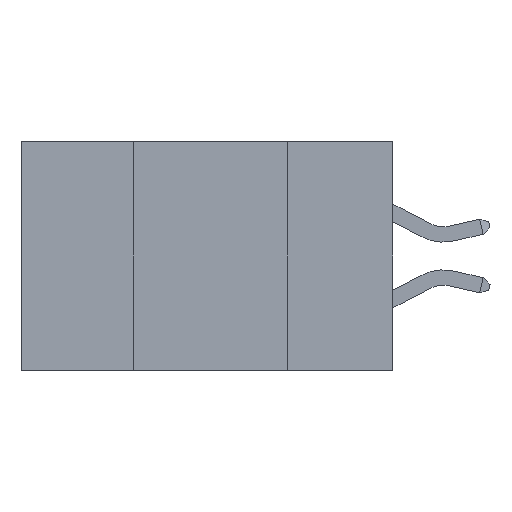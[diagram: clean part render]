
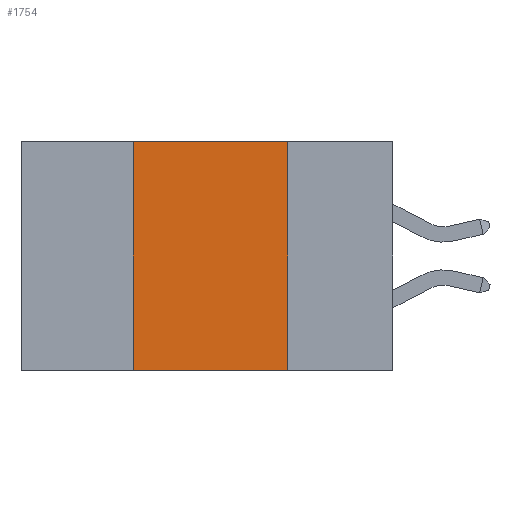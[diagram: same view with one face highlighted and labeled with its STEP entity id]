
A CAD part, left-side view. The second image highlights one B-rep face of the part: STEP entity #1754.
In plain terms, the highlighted planar face has unit normal (-1, 0, 0).
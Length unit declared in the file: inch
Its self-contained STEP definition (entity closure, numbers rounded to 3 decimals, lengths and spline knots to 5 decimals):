
#548 = VERTEX_POINT ( 'NONE', #22426 ) ;
#1312 = VERTEX_POINT ( 'NONE', #13641 ) ;
#1754 = ADVANCED_FACE ( 'NONE', ( #19253 ), #16965, .F. ) ;
#1822 = LINE ( 'NONE', #13468, #23692 ) ;
#3491 = ORIENTED_EDGE ( 'NONE', *, *, #4178, .T. ) ;
#3671 = DIRECTION ( 'NONE',  ( 1., 0., 0. ) ) ;
#3933 = ORIENTED_EDGE ( 'NONE', *, *, #21550, .F. ) ;
#4178 = EDGE_CURVE ( 'NONE', #20397, #548, #6258, .T. ) ;
#4592 = CARTESIAN_POINT ( 'NONE',  ( 0., 0.6, 0. ) ) ;
#5286 = EDGE_LOOP ( 'NONE', ( #19949, #3933, #6176, #3491 ) ) ;
#6176 = ORIENTED_EDGE ( 'NONE', *, *, #24717, .F. ) ;
#6258 = LINE ( 'NONE', #22367, #27716 ) ;
#7966 = DIRECTION ( 'NONE',  ( 0., 0., -1. ) ) ;
#8529 = LINE ( 'NONE', #18226, #10620 ) ;
#10620 = VECTOR ( 'NONE', #20649, 39.37008 ) ;
#11295 = DIRECTION ( 'NONE',  ( 0., -1., 0. ) ) ;
#13468 = CARTESIAN_POINT ( 'NONE',  ( 0., 0.42, 0. ) ) ;
#13641 = CARTESIAN_POINT ( 'NONE',  ( 0., 0.17, 0. ) ) ;
#13705 = CARTESIAN_POINT ( 'NONE',  ( 0., 0.42, -0.37 ) ) ;
#14936 = CARTESIAN_POINT ( 'NONE',  ( 0., 0.6, 0. ) ) ;
#16347 = VECTOR ( 'NONE', #11295, 39.37008 ) ;
#16682 = VERTEX_POINT ( 'NONE', #16713 ) ;
#16713 = CARTESIAN_POINT ( 'NONE',  ( 0., 0.42, 0. ) ) ;
#16965 = PLANE ( 'NONE',  #17863 ) ;
#17863 = AXIS2_PLACEMENT_3D ( 'NONE', #14936, #3671, #7966 ) ;
#18226 = CARTESIAN_POINT ( 'NONE',  ( 0., 0.17, 0. ) ) ;
#19253 = FACE_OUTER_BOUND ( 'NONE', #5286, .T. ) ;
#19949 = ORIENTED_EDGE ( 'NONE', *, *, #23741, .F. ) ;
#20397 = VERTEX_POINT ( 'NONE', #13705 ) ;
#20431 = DIRECTION ( 'NONE',  ( 0., 0., 1. ) ) ;
#20649 = DIRECTION ( 'NONE',  ( 0., 0., -1. ) ) ;
#21550 = EDGE_CURVE ( 'NONE', #16682, #1312, #24272, .T. ) ;
#22367 = CARTESIAN_POINT ( 'NONE',  ( 0., 0.6, -0.37 ) ) ;
#22426 = CARTESIAN_POINT ( 'NONE',  ( 0., 0.17, -0.37 ) ) ;
#23692 = VECTOR ( 'NONE', #20431, 39.37008 ) ;
#23741 = EDGE_CURVE ( 'NONE', #1312, #548, #8529, .T. ) ;
#24272 = LINE ( 'NONE', #4592, #16347 ) ;
#24557 = DIRECTION ( 'NONE',  ( 0., -1., 0. ) ) ;
#24717 = EDGE_CURVE ( 'NONE', #20397, #16682, #1822, .T. ) ;
#27716 = VECTOR ( 'NONE', #24557, 39.37008 ) ;
